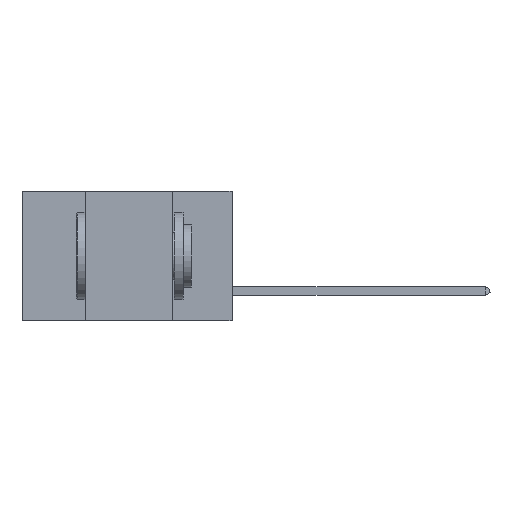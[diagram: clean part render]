
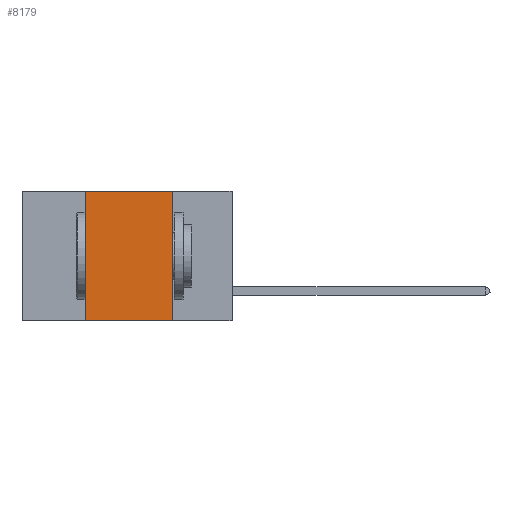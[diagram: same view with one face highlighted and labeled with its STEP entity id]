
A CAD part, left-side view. The second image highlights one B-rep face of the part: STEP entity #8179.
In plain terms, the highlighted planar face has unit normal (-1, 0, 0).
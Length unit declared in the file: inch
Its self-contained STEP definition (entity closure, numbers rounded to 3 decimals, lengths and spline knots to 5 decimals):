
#108 = DIRECTION ( 'NONE',  ( 0., -1., 0. ) ) ;
#690 = DIRECTION ( 'NONE',  ( 0., 0., -1. ) ) ;
#705 = VECTOR ( 'NONE', #108, 39.37008 ) ;
#1932 = AXIS2_PLACEMENT_3D ( 'NONE', #41732, #24696, #690 ) ;
#2487 = EDGE_LOOP ( 'NONE', ( #4091, #7247, #8063, #15649 ) ) ;
#3093 = VERTEX_POINT ( 'NONE', #11700 ) ;
#3549 = PLANE ( 'NONE',  #1932 ) ;
#4091 = ORIENTED_EDGE ( 'NONE', *, *, #14601, .F. ) ;
#7247 = ORIENTED_EDGE ( 'NONE', *, *, #8875, .F. ) ;
#8063 = ORIENTED_EDGE ( 'NONE', *, *, #44724, .F. ) ;
#8179 = ADVANCED_FACE ( 'NONE', ( #8604 ), #3549, .F. ) ;
#8604 = FACE_OUTER_BOUND ( 'NONE', #2487, .T. ) ;
#8875 = EDGE_CURVE ( 'NONE', #24774, #13689, #29606, .T. ) ;
#9544 = CARTESIAN_POINT ( 'NONE',  ( 0., 0.17, 0. ) ) ;
#11700 = CARTESIAN_POINT ( 'NONE',  ( 0., 0.42, -0.37 ) ) ;
#11774 = CARTESIAN_POINT ( 'NONE',  ( 0., 0.42, 0. ) ) ;
#13115 = LINE ( 'NONE', #34790, #705 ) ;
#13622 = LINE ( 'NONE', #9544, #18497 ) ;
#13689 = VERTEX_POINT ( 'NONE', #21398 ) ;
#14601 = EDGE_CURVE ( 'NONE', #13689, #28959, #13622, .T. ) ;
#14772 = DIRECTION ( 'NONE',  ( 0., -1., 0. ) ) ;
#15526 = DIRECTION ( 'NONE',  ( 0., 0., 1. ) ) ;
#15649 = ORIENTED_EDGE ( 'NONE', *, *, #31673, .T. ) ;
#16488 = DIRECTION ( 'NONE',  ( 0., 0., -1. ) ) ;
#18497 = VECTOR ( 'NONE', #16488, 39.37008 ) ;
#18899 = CARTESIAN_POINT ( 'NONE',  ( 0., 0.42, 0. ) ) ;
#21398 = CARTESIAN_POINT ( 'NONE',  ( 0., 0.17, 0. ) ) ;
#24696 = DIRECTION ( 'NONE',  ( 1., 0., 0. ) ) ;
#24774 = VERTEX_POINT ( 'NONE', #18899 ) ;
#28959 = VERTEX_POINT ( 'NONE', #35067 ) ;
#29606 = LINE ( 'NONE', #42538, #34401 ) ;
#31177 = LINE ( 'NONE', #11774, #38176 ) ;
#31673 = EDGE_CURVE ( 'NONE', #3093, #28959, #13115, .T. ) ;
#34401 = VECTOR ( 'NONE', #14772, 39.37008 ) ;
#34790 = CARTESIAN_POINT ( 'NONE',  ( 0., 0.6, -0.37 ) ) ;
#35067 = CARTESIAN_POINT ( 'NONE',  ( 0., 0.17, -0.37 ) ) ;
#38176 = VECTOR ( 'NONE', #15526, 39.37008 ) ;
#41732 = CARTESIAN_POINT ( 'NONE',  ( 0., 0.6, 0. ) ) ;
#42538 = CARTESIAN_POINT ( 'NONE',  ( 0., 0.6, 0. ) ) ;
#44724 = EDGE_CURVE ( 'NONE', #3093, #24774, #31177, .T. ) ;
